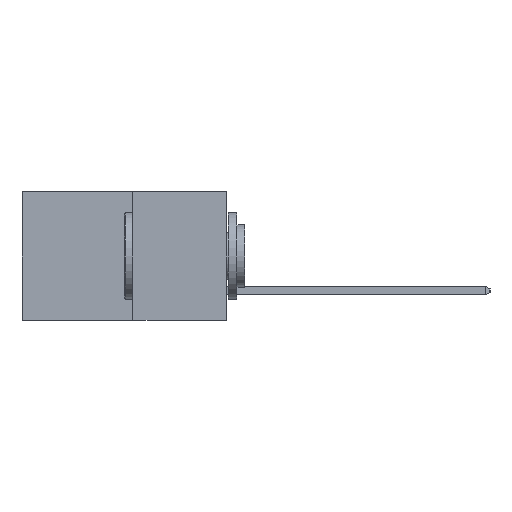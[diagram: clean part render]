
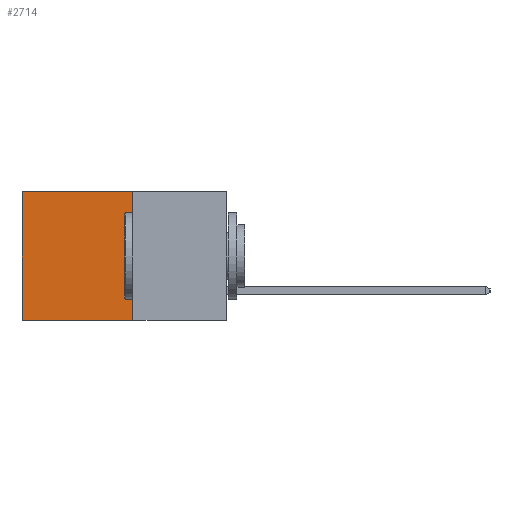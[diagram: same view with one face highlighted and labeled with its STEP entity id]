
A CAD part, left-side view. The second image highlights one B-rep face of the part: STEP entity #2714.
In plain terms, the highlighted planar face has unit normal (-1, 0, 0).
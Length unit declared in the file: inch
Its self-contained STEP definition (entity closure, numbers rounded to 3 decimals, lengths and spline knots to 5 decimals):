
#939 = VECTOR ( 'NONE', #11966, 39.37008 ) ;
#1291 = EDGE_CURVE ( 'NONE', #11307, #10352, #6123, .T. ) ;
#1383 = VERTEX_POINT ( 'NONE', #4669 ) ;
#1479 = ORIENTED_EDGE ( 'NONE', *, *, #9860, .T. ) ;
#2631 = CARTESIAN_POINT ( 'NONE',  ( 0.277, 0.27, 0. ) ) ;
#2654 = DIRECTION ( 'NONE',  ( 0., 0., -1. ) ) ;
#2686 = PLANE ( 'NONE',  #4847 ) ;
#2714 = ADVANCED_FACE ( 'NONE', ( #6390 ), #2686, .F. ) ;
#3175 = CARTESIAN_POINT ( 'NONE',  ( 0.277, 0.27, 0. ) ) ;
#3322 = ORIENTED_EDGE ( 'NONE', *, *, #6453, .T. ) ;
#3579 = VECTOR ( 'NONE', #6632, 39.37008 ) ;
#3897 = CARTESIAN_POINT ( 'NONE',  ( 0.277, 0.59, -0.37 ) ) ;
#4669 = CARTESIAN_POINT ( 'NONE',  ( 0.277, 0.59, 0. ) ) ;
#4735 = VECTOR ( 'NONE', #11439, 39.37008 ) ;
#4776 = ORIENTED_EDGE ( 'NONE', *, *, #1291, .F. ) ;
#4847 = AXIS2_PLACEMENT_3D ( 'NONE', #12076, #11205, #2654 ) ;
#5021 = LINE ( 'NONE', #3175, #4735 ) ;
#5692 = EDGE_CURVE ( 'NONE', #10352, #10475, #11590, .T. ) ;
#5751 = LINE ( 'NONE', #3897, #3579 ) ;
#6123 = LINE ( 'NONE', #9626, #939 ) ;
#6260 = ORIENTED_EDGE ( 'NONE', *, *, #5692, .F. ) ;
#6390 = FACE_OUTER_BOUND ( 'NONE', #9239, .T. ) ;
#6453 = EDGE_CURVE ( 'NONE', #1383, #10475, #5751, .T. ) ;
#6529 = CARTESIAN_POINT ( 'NONE',  ( 0.277, 0.27, -0.37 ) ) ;
#6632 = DIRECTION ( 'NONE',  ( 0., 0., -1. ) ) ;
#7760 = CARTESIAN_POINT ( 'NONE',  ( 0.277, 0.27, -0.37 ) ) ;
#7958 = CARTESIAN_POINT ( 'NONE',  ( 0.277, 0.59, -0.37 ) ) ;
#9199 = VECTOR ( 'NONE', #9279, 39.37008 ) ;
#9239 = EDGE_LOOP ( 'NONE', ( #3322, #6260, #4776, #1479 ) ) ;
#9279 = DIRECTION ( 'NONE',  ( 0., 1., 0. ) ) ;
#9626 = CARTESIAN_POINT ( 'NONE',  ( 0.277, 0.27, -0.37 ) ) ;
#9860 = EDGE_CURVE ( 'NONE', #11307, #1383, #5021, .T. ) ;
#10352 = VERTEX_POINT ( 'NONE', #7760 ) ;
#10475 = VERTEX_POINT ( 'NONE', #7958 ) ;
#11205 = DIRECTION ( 'NONE',  ( 1., 0., 0. ) ) ;
#11307 = VERTEX_POINT ( 'NONE', #2631 ) ;
#11439 = DIRECTION ( 'NONE',  ( 0., 1., 0. ) ) ;
#11590 = LINE ( 'NONE', #6529, #9199 ) ;
#11966 = DIRECTION ( 'NONE',  ( 0., 0., -1. ) ) ;
#12076 = CARTESIAN_POINT ( 'NONE',  ( 0.277, 0.27, -0.37 ) ) ;
